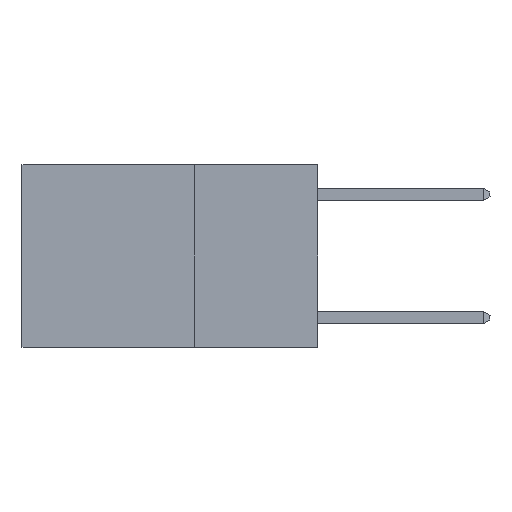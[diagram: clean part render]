
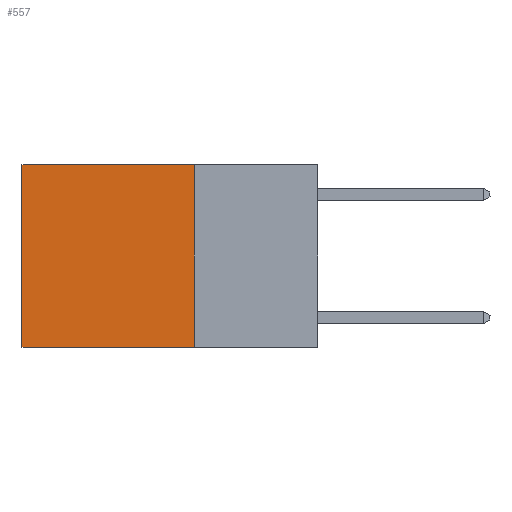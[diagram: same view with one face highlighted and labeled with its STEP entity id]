
A CAD part, left-side view. The second image highlights one B-rep face of the part: STEP entity #557.
In plain terms, the highlighted planar face has unit normal (-1, 0, 0).
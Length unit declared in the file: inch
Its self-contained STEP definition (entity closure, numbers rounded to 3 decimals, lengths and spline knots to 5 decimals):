
#372 = LINE ( 'NONE', #1057, #5288 ) ;
#382 = ORIENTED_EDGE ( 'NONE', *, *, #7811, .F. ) ;
#506 = CARTESIAN_POINT ( 'NONE',  ( 0.2625, 0.25, -0.37 ) ) ;
#557 = ADVANCED_FACE ( 'NONE', ( #3217 ), #6126, .F. ) ;
#1057 = CARTESIAN_POINT ( 'NONE',  ( 0.2625, 0.6, 0. ) ) ;
#1249 = EDGE_LOOP ( 'NONE', ( #6084, #7673, #382, #3706 ) ) ;
#1270 = CARTESIAN_POINT ( 'NONE',  ( 0.2625, 0.6, 0. ) ) ;
#1496 = DIRECTION ( 'NONE',  ( 0., 1., 0. ) ) ;
#1821 = EDGE_CURVE ( 'NONE', #5014, #6990, #372, .T. ) ;
#1955 = DIRECTION ( 'NONE',  ( 1., 0., 0. ) ) ;
#2089 = EDGE_CURVE ( 'NONE', #7217, #6990, #8040, .T. ) ;
#2373 = EDGE_CURVE ( 'NONE', #5242, #5014, #8804, .T. ) ;
#3007 = DIRECTION ( 'NONE',  ( 0., 0., -1. ) ) ;
#3217 = FACE_OUTER_BOUND ( 'NONE', #1249, .T. ) ;
#3373 = VECTOR ( 'NONE', #7882, 39.37008 ) ;
#3706 = ORIENTED_EDGE ( 'NONE', *, *, #2373, .T. ) ;
#3802 = VECTOR ( 'NONE', #8764, 39.37008 ) ;
#4302 = CARTESIAN_POINT ( 'NONE',  ( 0.2625, 0.25, 0. ) ) ;
#4609 = CARTESIAN_POINT ( 'NONE',  ( 0.2625, 0.25, 0. ) ) ;
#5014 = VERTEX_POINT ( 'NONE', #1270 ) ;
#5242 = VERTEX_POINT ( 'NONE', #4609 ) ;
#5288 = VECTOR ( 'NONE', #3007, 39.37008 ) ;
#6084 = ORIENTED_EDGE ( 'NONE', *, *, #1821, .T. ) ;
#6126 = PLANE ( 'NONE',  #7770 ) ;
#6137 = CARTESIAN_POINT ( 'NONE',  ( 0.2625, 0.25, 0. ) ) ;
#6322 = DIRECTION ( 'NONE',  ( 0., 0., -1. ) ) ;
#6445 = LINE ( 'NONE', #4302, #3373 ) ;
#6786 = CARTESIAN_POINT ( 'NONE',  ( 0.2625, 0.6, -0.37 ) ) ;
#6990 = VERTEX_POINT ( 'NONE', #6786 ) ;
#7125 = VECTOR ( 'NONE', #1496, 39.37008 ) ;
#7217 = VERTEX_POINT ( 'NONE', #506 ) ;
#7673 = ORIENTED_EDGE ( 'NONE', *, *, #2089, .F. ) ;
#7770 = AXIS2_PLACEMENT_3D ( 'NONE', #8426, #1955, #6322 ) ;
#7811 = EDGE_CURVE ( 'NONE', #5242, #7217, #6445, .T. ) ;
#7882 = DIRECTION ( 'NONE',  ( 0., 0., -1. ) ) ;
#8040 = LINE ( 'NONE', #9289, #7125 ) ;
#8426 = CARTESIAN_POINT ( 'NONE',  ( 0.2625, 0.25, 0. ) ) ;
#8764 = DIRECTION ( 'NONE',  ( 0., 1., 0. ) ) ;
#8804 = LINE ( 'NONE', #6137, #3802 ) ;
#9289 = CARTESIAN_POINT ( 'NONE',  ( 0.2625, 0.25, -0.37 ) ) ;
